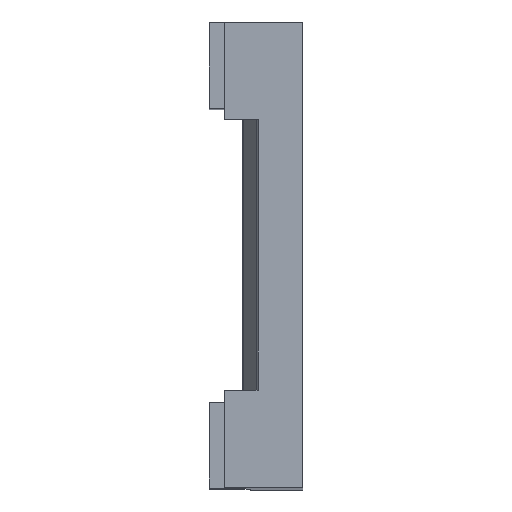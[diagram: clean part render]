
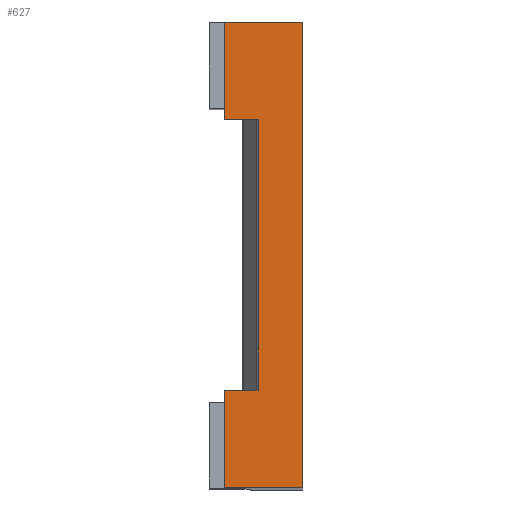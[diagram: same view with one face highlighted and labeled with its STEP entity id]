
A CAD part, top view. The second image highlights one B-rep face of the part: STEP entity #627.
In plain terms, the highlighted planar face has unit normal (0, 0, 1).
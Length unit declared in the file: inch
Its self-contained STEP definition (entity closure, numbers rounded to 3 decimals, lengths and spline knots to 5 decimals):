
#25=PLANE('',#685);
#53=FACE_OUTER_BOUND('',#89,.T.);
#89=EDGE_LOOP('',(#475,#476,#477,#478,#479,#480,#481,#482));
#125=LINE('',#919,#199);
#127=LINE('',#923,#201);
#140=LINE('',#957,#214);
#141=LINE('',#959,#215);
#142=LINE('',#961,#216);
#143=LINE('',#963,#217);
#144=LINE('',#965,#218);
#145=LINE('',#966,#219);
#199=VECTOR('',#749,0.3937);
#201=VECTOR('',#753,0.3937);
#214=VECTOR('',#776,0.3937);
#215=VECTOR('',#777,0.3937);
#216=VECTOR('',#778,0.3937);
#217=VECTOR('',#779,0.3937);
#218=VECTOR('',#780,0.3937);
#219=VECTOR('',#781,0.3937);
#293=VERTEX_POINT('',#916);
#294=VERTEX_POINT('',#918);
#295=VERTEX_POINT('',#922);
#311=VERTEX_POINT('',#956);
#312=VERTEX_POINT('',#958);
#313=VERTEX_POINT('',#960);
#314=VERTEX_POINT('',#962);
#315=VERTEX_POINT('',#964);
#357=EDGE_CURVE('',#294,#293,#125,.T.);
#359=EDGE_CURVE('',#294,#295,#127,.T.);
#376=EDGE_CURVE('',#293,#311,#140,.T.);
#377=EDGE_CURVE('',#311,#312,#141,.T.);
#378=EDGE_CURVE('',#313,#312,#142,.T.);
#379=EDGE_CURVE('',#313,#314,#143,.T.);
#380=EDGE_CURVE('',#314,#315,#144,.T.);
#381=EDGE_CURVE('',#315,#295,#145,.T.);
#475=ORIENTED_EDGE('',*,*,#357,.T.);
#476=ORIENTED_EDGE('',*,*,#376,.T.);
#477=ORIENTED_EDGE('',*,*,#377,.T.);
#478=ORIENTED_EDGE('',*,*,#378,.F.);
#479=ORIENTED_EDGE('',*,*,#379,.T.);
#480=ORIENTED_EDGE('',*,*,#380,.T.);
#481=ORIENTED_EDGE('',*,*,#381,.T.);
#482=ORIENTED_EDGE('',*,*,#359,.F.);
#627=ADVANCED_FACE('',(#53),#25,.T.);
#685=AXIS2_PLACEMENT_3D('',#955,#774,#775);
#749=DIRECTION('',(0.,1.,0.));
#753=DIRECTION('',(-1.,0.,0.));
#774=DIRECTION('center_axis',(0.,0.,1.));
#775=DIRECTION('ref_axis',(-1.,0.,0.));
#776=DIRECTION('',(-1.,0.,0.));
#777=DIRECTION('',(0.,-1.,0.));
#778=DIRECTION('',(-1.,0.,0.));
#779=DIRECTION('',(0.,-1.,0.));
#780=DIRECTION('',(-1.,0.,0.));
#781=DIRECTION('',(0.,-1.,0.));
#916=CARTESIAN_POINT('',(-0.34519,0.23622,3.3807));
#918=CARTESIAN_POINT('',(-0.34519,-1.00422,3.3807));
#919=CARTESIAN_POINT('',(-0.34519,-0.07389,3.3807));
#922=CARTESIAN_POINT('',(-0.55475,-1.00422,3.3807));
#923=CARTESIAN_POINT('',(-0.24878,-1.00422,3.3807));
#955=CARTESIAN_POINT('Origin',(-0.24878,0.23622,3.3807));
#956=CARTESIAN_POINT('',(-0.55475,0.23622,3.3807));
#957=CARTESIAN_POINT('',(-0.24878,0.23622,3.3807));
#958=CARTESIAN_POINT('',(-0.55475,-0.02313,3.3807));
#959=CARTESIAN_POINT('',(-0.55475,-0.20356,3.3807));
#960=CARTESIAN_POINT('',(-0.46475,-0.02313,3.3807));
#961=CARTESIAN_POINT('',(-0.24878,-0.02313,3.3807));
#962=CARTESIAN_POINT('',(-0.46475,-0.74487,3.3807));
#963=CARTESIAN_POINT('',(-0.46475,0.23622,3.3807));
#964=CARTESIAN_POINT('',(-0.55475,-0.74487,3.3807));
#965=CARTESIAN_POINT('',(-0.24878,-0.74487,3.3807));
#966=CARTESIAN_POINT('',(-0.55475,-0.69411,3.3807));
